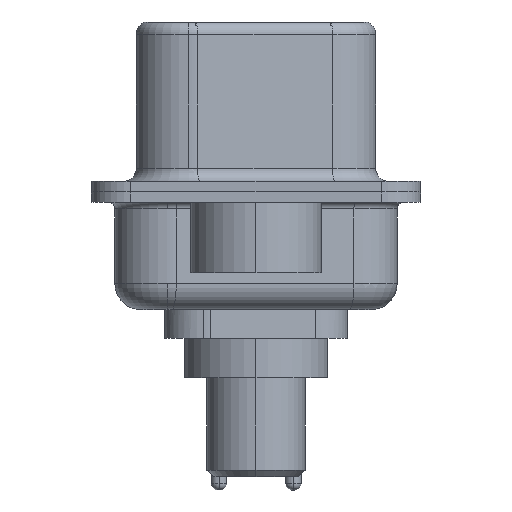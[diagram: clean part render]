
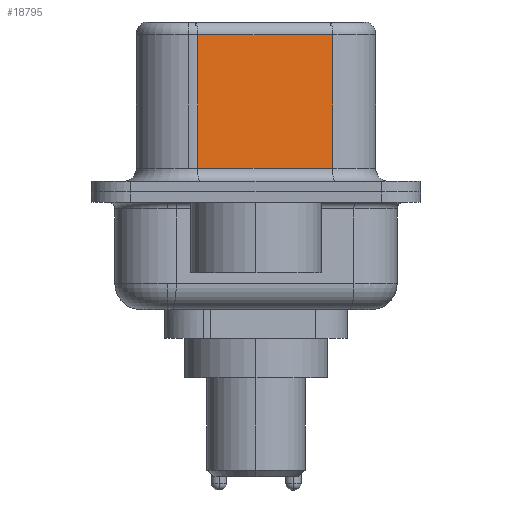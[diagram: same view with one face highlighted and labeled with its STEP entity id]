
A CAD part, left-side view. The second image highlights one B-rep face of the part: STEP entity #18795.
In plain terms, the highlighted planar face has unit normal (-0.985, -0.174, 0).
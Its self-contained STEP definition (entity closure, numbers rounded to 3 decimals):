
#329 = LINE ( 'NONE', #1027, #25143 ) ;
#1027 = CARTESIAN_POINT ( 'NONE',  ( 4.58, -2.927, 6.52 ) ) ;
#1295 = LINE ( 'NONE', #9849, #11063 ) ;
#1422 = PLANE ( 'NONE',  #21415 ) ;
#1584 = ORIENTED_EDGE ( 'NONE', *, *, #3486, .T. ) ;
#1614 = CARTESIAN_POINT ( 'NONE',  ( 3.67, 2.233, 6.52 ) ) ;
#1862 = CARTESIAN_POINT ( 'NONE',  ( 3.67, 2.233, 0.9 ) ) ;
#2145 = ORIENTED_EDGE ( 'NONE', *, *, #2335, .T. ) ;
#2335 = EDGE_CURVE ( 'NONE', #11471, #11213, #3171, .T. ) ;
#3171 = LINE ( 'NONE', #1614, #12923 ) ;
#3384 = VECTOR ( 'NONE', #10722, 1000. ) ;
#3486 = EDGE_CURVE ( 'NONE', #4752, #11471, #1295, .T. ) ;
#3527 = DIRECTION ( 'NONE',  ( -0.174, 0.985, 0. ) ) ;
#4640 = CARTESIAN_POINT ( 'NONE',  ( 4.58, -2.927, 0.9 ) ) ;
#4752 = VERTEX_POINT ( 'NONE', #24524 ) ;
#5375 = DIRECTION ( 'NONE',  ( 0.985, 0.174, 0. ) ) ;
#9159 = FACE_OUTER_BOUND ( 'NONE', #14834, .T. ) ;
#9849 = CARTESIAN_POINT ( 'NONE',  ( 4.58, -2.927, 6.02 ) ) ;
#10722 = DIRECTION ( 'NONE',  ( 0.174, -0.985, 0. ) ) ;
#11063 = VECTOR ( 'NONE', #3527, 1000. ) ;
#11213 = VERTEX_POINT ( 'NONE', #1862 ) ;
#11471 = VERTEX_POINT ( 'NONE', #14103 ) ;
#12923 = VECTOR ( 'NONE', #25100, 1000. ) ;
#13125 = LINE ( 'NONE', #24481, #3384 ) ;
#14103 = CARTESIAN_POINT ( 'NONE',  ( 3.67, 2.233, 6.02 ) ) ;
#14834 = EDGE_LOOP ( 'NONE', ( #18427, #1584, #2145, #24973 ) ) ;
#15050 = CARTESIAN_POINT ( 'NONE',  ( 4.58, -2.927, 6.52 ) ) ;
#16100 = VERTEX_POINT ( 'NONE', #4640 ) ;
#17407 = EDGE_CURVE ( 'NONE', #11213, #16100, #13125, .T. ) ;
#18427 = ORIENTED_EDGE ( 'NONE', *, *, #19012, .F. ) ;
#18795 = ADVANCED_FACE ( 'NONE', ( #9159 ), #1422, .F. ) ;
#19012 = EDGE_CURVE ( 'NONE', #4752, #16100, #329, .T. ) ;
#19027 = DIRECTION ( 'NONE',  ( -0.174, 0.985, 0. ) ) ;
#21415 = AXIS2_PLACEMENT_3D ( 'NONE', #15050, #5375, #19027 ) ;
#22538 = DIRECTION ( 'NONE',  ( 0., 0., -1. ) ) ;
#24481 = CARTESIAN_POINT ( 'NONE',  ( 4.58, -2.927, 0.9 ) ) ;
#24524 = CARTESIAN_POINT ( 'NONE',  ( 4.58, -2.927, 6.02 ) ) ;
#24973 = ORIENTED_EDGE ( 'NONE', *, *, #17407, .T. ) ;
#25100 = DIRECTION ( 'NONE',  ( 0., 0., -1. ) ) ;
#25143 = VECTOR ( 'NONE', #22538, 1000. ) ;
